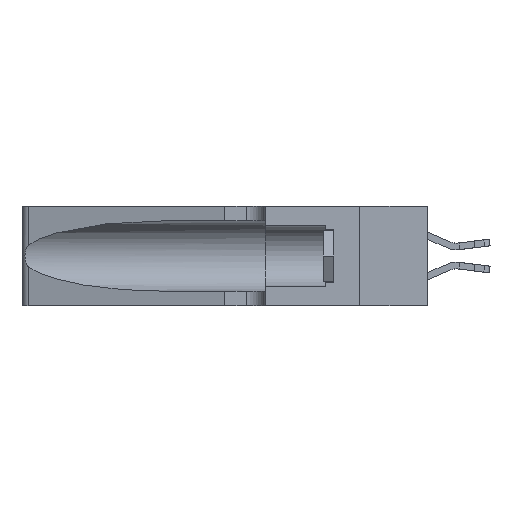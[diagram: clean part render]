
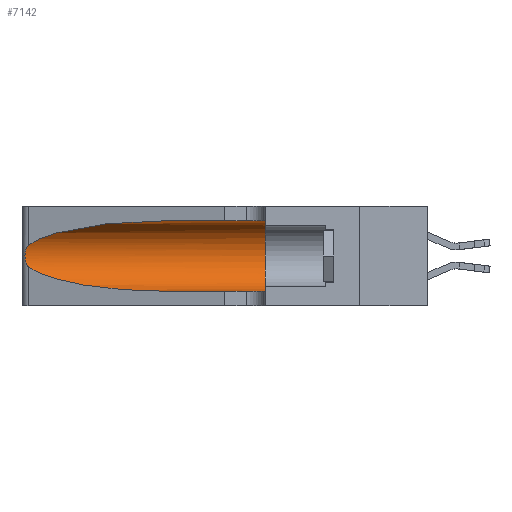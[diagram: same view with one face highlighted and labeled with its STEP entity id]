
A CAD part, left-side view. The second image highlights one B-rep face of the part: STEP entity #7142.
In plain terms, the highlighted cylindrical face has radius 3.308 mm (diameter 6.617 mm), a partial arc.
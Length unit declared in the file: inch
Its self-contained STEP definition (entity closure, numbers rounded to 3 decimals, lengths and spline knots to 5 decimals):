
#56 = CARTESIAN_POINT ( 'NONE',  ( 0.1305, 0.72297, 0.05475 ) ) ;
#386 = ORIENTED_EDGE ( 'NONE', *, *, #25111, .T. ) ;
#704 = CARTESIAN_POINT ( 'NONE',  ( 0.1305, 0.72297, 0.31525 ) ) ;
#821 =( BOUNDED_CURVE ( )  B_SPLINE_CURVE ( 3, ( #7687, #1513, #17556, #5705 ),
 .UNSPECIFIED., .F., .T. ) 
 B_SPLINE_CURVE_WITH_KNOTS ( ( 4, 4 ),
 ( 1.5708, 2.84003 ),
 .UNSPECIFIED. ) 
 CURVE ( )  GEOMETRIC_REPRESENTATION_ITEM ( )  RATIONAL_B_SPLINE_CURVE ( ( 1., 0.87, 0.87, 1. ) ) 
 REPRESENTATION_ITEM ( '' )  );
#900 = CARTESIAN_POINT ( 'NONE',  ( 0.1305, 1.61858, 0.185 ) ) ;
#1262 = CARTESIAN_POINT ( 'NONE',  ( 0.1305, 0.35, 0.31525 ) ) ;
#1513 = CARTESIAN_POINT ( 'NONE',  ( 0.18966, 0.96281, 0.31525 ) ) ;
#1766 = CARTESIAN_POINT ( 'NONE',  ( 0.1305, 1.61858, 0.05475 ) ) ;
#2269 = EDGE_CURVE ( 'NONE', #14022, #13453, #4839, .T. ) ;
#3871 = DIRECTION ( 'NONE',  ( 0., -1., 0. ) ) ;
#3911 = CARTESIAN_POINT ( 'NONE',  ( 0.1305, 1.61858, 0.31525 ) ) ;
#4030 =( BOUNDED_CURVE ( )  B_SPLINE_CURVE ( 3, ( #10786, #18676, #6894, #20629 ),
 .UNSPECIFIED., .F., .T. ) 
 B_SPLINE_CURVE_WITH_KNOTS ( ( 4, 4 ),
 ( 3.44316, 4.71239 ),
 .UNSPECIFIED. ) 
 CURVE ( )  GEOMETRIC_REPRESENTATION_ITEM ( )  RATIONAL_B_SPLINE_CURVE ( ( 1., 0.87, 0.87, 1. ) ) 
 REPRESENTATION_ITEM ( '' )  );
#4088 = CARTESIAN_POINT ( 'NONE',  ( 0.26018, 1.23835, 0.19895 ) ) ;
#4215 = CARTESIAN_POINT ( 'NONE',  ( 0.25639, 1.23186, 0.15144 ) ) ;
#4839 = B_SPLINE_CURVE_WITH_KNOTS ( 'NONE', 3,
 ( #15854, #21386, #22874, #8096, #6798, #4088, #9163, #8375, #8241, #7182, #7411, #4215, #21475, #15228 ),
 .UNSPECIFIED., .F., .F.,
 ( 4, 2, 2, 2, 2, 2, 4 ),
 ( 0., 0.00027, 0.00053, 0.00107, 0.0016, 0.00187, 0.00214 ),
 .UNSPECIFIED. ) ;
#5415 = EDGE_CURVE ( 'NONE', #13453, #8838, #4030, .T. ) ;
#5705 = CARTESIAN_POINT ( 'NONE',  ( 0.25487, 1.22718, 0.22369 ) ) ;
#6635 = AXIS2_PLACEMENT_3D ( 'NONE', #19382, #7626, #21314 ) ;
#6798 = CARTESIAN_POINT ( 'NONE',  ( 0.25854, 1.2359, 0.20912 ) ) ;
#6894 = CARTESIAN_POINT ( 'NONE',  ( 0.18966, 0.96281, 0.05475 ) ) ;
#7142 = ADVANCED_FACE ( 'NONE', ( #11388 ), #21194, .F. ) ;
#7182 = CARTESIAN_POINT ( 'NONE',  ( 0.25856, 1.23593, 0.16098 ) ) ;
#7411 = CARTESIAN_POINT ( 'NONE',  ( 0.25789, 1.23486, 0.15765 ) ) ;
#7626 = DIRECTION ( 'NONE',  ( 0., 1., 0. ) ) ;
#7687 = CARTESIAN_POINT ( 'NONE',  ( 0.1305, 0.72297, 0.31525 ) ) ;
#7988 = CARTESIAN_POINT ( 'NONE',  ( 0.25487, 1.22718, 0.22369 ) ) ;
#8096 = CARTESIAN_POINT ( 'NONE',  ( 0.25787, 1.23484, 0.2124 ) ) ;
#8241 = CARTESIAN_POINT ( 'NONE',  ( 0.26017, 1.23833, 0.17102 ) ) ;
#8375 = CARTESIAN_POINT ( 'NONE',  ( 0.26075, 1.23896, 0.178 ) ) ;
#8838 = VERTEX_POINT ( 'NONE', #56 ) ;
#9163 = CARTESIAN_POINT ( 'NONE',  ( 0.26075, 1.23896, 0.19203 ) ) ;
#9242 = DIRECTION ( 'NONE',  ( 0., -1., 0. ) ) ;
#9299 = VECTOR ( 'NONE', #23560, 39.37008 ) ;
#10786 = CARTESIAN_POINT ( 'NONE',  ( 0.25487, 1.22718, 0.14631 ) ) ;
#11355 = VECTOR ( 'NONE', #3871, 39.37008 ) ;
#11388 = FACE_OUTER_BOUND ( 'NONE', #16510, .T. ) ;
#13453 = VERTEX_POINT ( 'NONE', #22100 ) ;
#13984 = ORIENTED_EDGE ( 'NONE', *, *, #22584, .T. ) ;
#14022 = VERTEX_POINT ( 'NONE', #7988 ) ;
#14334 = VERTEX_POINT ( 'NONE', #704 ) ;
#14705 = EDGE_CURVE ( 'NONE', #14334, #17495, #24816, .T. ) ;
#15228 = CARTESIAN_POINT ( 'NONE',  ( 0.25487, 1.22718, 0.14631 ) ) ;
#15247 = ORIENTED_EDGE ( 'NONE', *, *, #5415, .T. ) ;
#15854 = CARTESIAN_POINT ( 'NONE',  ( 0.25487, 1.22718, 0.22369 ) ) ;
#16465 = ORIENTED_EDGE ( 'NONE', *, *, #20093, .F. ) ;
#16510 = EDGE_LOOP ( 'NONE', ( #13984, #24924, #15247, #386, #16465, #22246 ) ) ;
#17449 = CIRCLE ( 'NONE', #6635, 0.13025 ) ;
#17495 = VERTEX_POINT ( 'NONE', #1262 ) ;
#17556 = CARTESIAN_POINT ( 'NONE',  ( 0.2373, 1.15595, 0.28018 ) ) ;
#18676 = CARTESIAN_POINT ( 'NONE',  ( 0.2373, 1.15595, 0.08982 ) ) ;
#19382 = CARTESIAN_POINT ( 'NONE',  ( 0.1305, 0.35, 0.185 ) ) ;
#19478 = CARTESIAN_POINT ( 'NONE',  ( 0.1305, 0.35, 0.05475 ) ) ;
#20093 = EDGE_CURVE ( 'NONE', #17495, #25590, #17449, .T. ) ;
#20629 = CARTESIAN_POINT ( 'NONE',  ( 0.1305, 0.72297, 0.05475 ) ) ;
#20982 = DIRECTION ( 'NONE',  ( 0., 0., -1. ) ) ;
#21140 = AXIS2_PLACEMENT_3D ( 'NONE', #900, #9242, #20982 ) ;
#21194 = CYLINDRICAL_SURFACE ( 'NONE', #21140, 0.13025 ) ;
#21314 = DIRECTION ( 'NONE',  ( 0., 0., 1. ) ) ;
#21386 = CARTESIAN_POINT ( 'NONE',  ( 0.25555, 1.22994, 0.2215 ) ) ;
#21475 = CARTESIAN_POINT ( 'NONE',  ( 0.25555, 1.22993, 0.14849 ) ) ;
#22100 = CARTESIAN_POINT ( 'NONE',  ( 0.25487, 1.22718, 0.14631 ) ) ;
#22246 = ORIENTED_EDGE ( 'NONE', *, *, #14705, .F. ) ;
#22359 = LINE ( 'NONE', #1766, #11355 ) ;
#22584 = EDGE_CURVE ( 'NONE', #14334, #14022, #821, .T. ) ;
#22874 = CARTESIAN_POINT ( 'NONE',  ( 0.25639, 1.23184, 0.21858 ) ) ;
#23560 = DIRECTION ( 'NONE',  ( 0., -1., 0. ) ) ;
#24816 = LINE ( 'NONE', #3911, #9299 ) ;
#24924 = ORIENTED_EDGE ( 'NONE', *, *, #2269, .T. ) ;
#25111 = EDGE_CURVE ( 'NONE', #8838, #25590, #22359, .T. ) ;
#25590 = VERTEX_POINT ( 'NONE', #19478 ) ;
